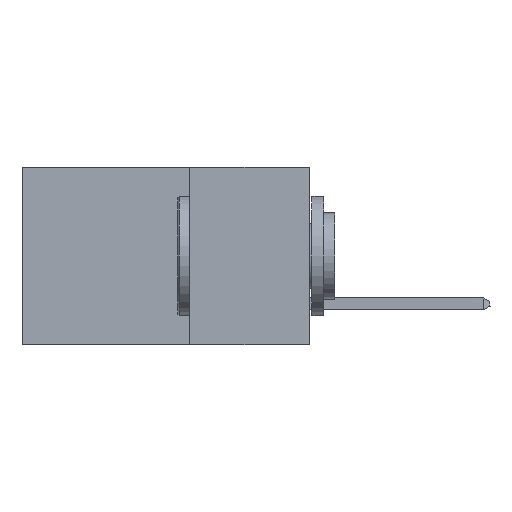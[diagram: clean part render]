
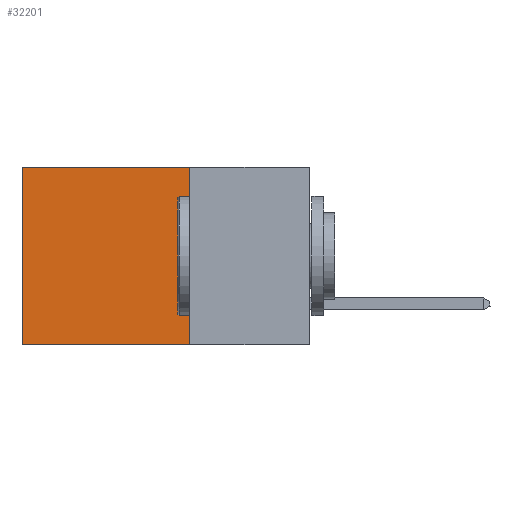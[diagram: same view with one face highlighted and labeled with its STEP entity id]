
A CAD part, left-side view. The second image highlights one B-rep face of the part: STEP entity #32201.
In plain terms, the highlighted planar face has unit normal (-1, 0, 0).
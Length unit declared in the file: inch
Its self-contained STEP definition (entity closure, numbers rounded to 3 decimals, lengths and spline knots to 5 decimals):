
#473 = LINE ( 'NONE', #28206, #19001 ) ;
#2724 = CARTESIAN_POINT ( 'NONE',  ( 0.2875, 0.25, 0. ) ) ;
#5456 = VECTOR ( 'NONE', #21215, 39.37008 ) ;
#7967 = EDGE_CURVE ( 'NONE', #11611, #31664, #473, .T. ) ;
#11611 = VERTEX_POINT ( 'NONE', #30489 ) ;
#12911 = EDGE_CURVE ( 'NONE', #45274, #46174, #14041, .T. ) ;
#14041 = LINE ( 'NONE', #2724, #28697 ) ;
#14393 = ORIENTED_EDGE ( 'NONE', *, *, #45964, .T. ) ;
#15024 = CARTESIAN_POINT ( 'NONE',  ( 0.2875, 0.25, -0.37 ) ) ;
#15124 = VECTOR ( 'NONE', #45765, 39.37008 ) ;
#17286 = DIRECTION ( 'NONE',  ( 0., 0., -1. ) ) ;
#19001 = VECTOR ( 'NONE', #43638, 39.37008 ) ;
#19166 = DIRECTION ( 'NONE',  ( 0., 0., -1. ) ) ;
#19744 = CARTESIAN_POINT ( 'NONE',  ( 0.2875, 0.6, -0.37 ) ) ;
#20354 = CARTESIAN_POINT ( 'NONE',  ( 0.2875, 0.25, 0. ) ) ;
#20962 = CARTESIAN_POINT ( 'NONE',  ( 0.2875, 0.25, -0.37 ) ) ;
#21215 = DIRECTION ( 'NONE',  ( 0., 1., 0. ) ) ;
#21658 = ORIENTED_EDGE ( 'NONE', *, *, #22922, .F. ) ;
#22235 = AXIS2_PLACEMENT_3D ( 'NONE', #44271, #30049, #19166 ) ;
#22922 = EDGE_CURVE ( 'NONE', #46174, #31664, #23016, .T. ) ;
#23016 = LINE ( 'NONE', #20962, #15124 ) ;
#26054 = FACE_OUTER_BOUND ( 'NONE', #42984, .T. ) ;
#28206 = CARTESIAN_POINT ( 'NONE',  ( 0.2875, 0.6, 0. ) ) ;
#28697 = VECTOR ( 'NONE', #17286, 39.37008 ) ;
#30049 = DIRECTION ( 'NONE',  ( 1., 0., 0. ) ) ;
#30489 = CARTESIAN_POINT ( 'NONE',  ( 0.2875, 0.6, 0. ) ) ;
#30779 = LINE ( 'NONE', #45716, #5456 ) ;
#31664 = VERTEX_POINT ( 'NONE', #19744 ) ;
#32201 = ADVANCED_FACE ( 'NONE', ( #26054 ), #33979, .F. ) ;
#33979 = PLANE ( 'NONE',  #22235 ) ;
#42156 = ORIENTED_EDGE ( 'NONE', *, *, #7967, .T. ) ;
#42984 = EDGE_LOOP ( 'NONE', ( #42156, #21658, #46135, #14393 ) ) ;
#43638 = DIRECTION ( 'NONE',  ( 0., 0., -1. ) ) ;
#44271 = CARTESIAN_POINT ( 'NONE',  ( 0.2875, 0.25, 0. ) ) ;
#45274 = VERTEX_POINT ( 'NONE', #20354 ) ;
#45716 = CARTESIAN_POINT ( 'NONE',  ( 0.2875, 0.25, 0. ) ) ;
#45765 = DIRECTION ( 'NONE',  ( 0., 1., 0. ) ) ;
#45964 = EDGE_CURVE ( 'NONE', #45274, #11611, #30779, .T. ) ;
#46135 = ORIENTED_EDGE ( 'NONE', *, *, #12911, .F. ) ;
#46174 = VERTEX_POINT ( 'NONE', #15024 ) ;
